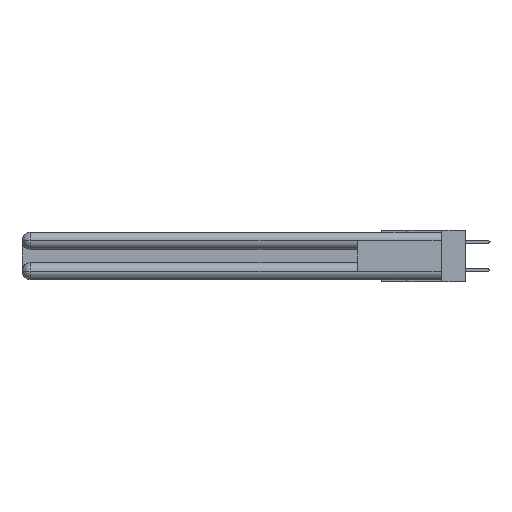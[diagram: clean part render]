
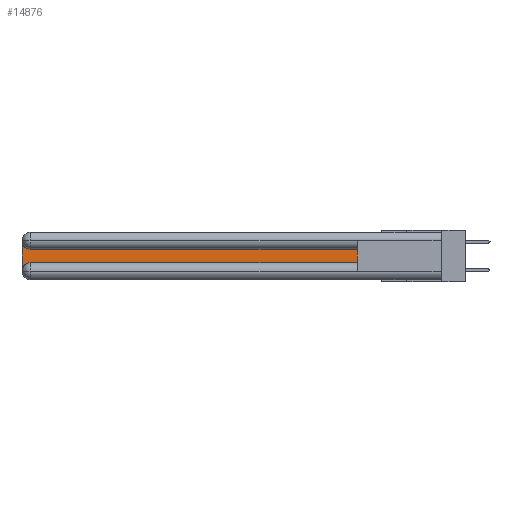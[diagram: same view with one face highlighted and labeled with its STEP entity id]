
A CAD part, left-side view. The second image highlights one B-rep face of the part: STEP entity #14876.
In plain terms, the highlighted planar face has unit normal (-1, 0, 0).
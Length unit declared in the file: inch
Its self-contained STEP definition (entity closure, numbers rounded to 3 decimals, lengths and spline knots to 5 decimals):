
#285 = ORIENTED_EDGE ( 'NONE', *, *, #8577, .T. ) ;
#614 = LINE ( 'NONE', #4832, #23441 ) ;
#1921 = CARTESIAN_POINT ( 'NONE',  ( 0.075, 0.6, -0.2175 ) ) ;
#2613 = VERTEX_POINT ( 'NONE', #20632 ) ;
#2625 = EDGE_CURVE ( 'NONE', #20399, #27930, #19876, .T. ) ;
#2728 = VECTOR ( 'NONE', #16100, 39.37008 ) ;
#3406 = LINE ( 'NONE', #16903, #12643 ) ;
#3561 = CARTESIAN_POINT ( 'NONE',  ( 0.075, 3., -0.2775 ) ) ;
#3810 = LINE ( 'NONE', #11492, #13066 ) ;
#4277 = DIRECTION ( 'NONE',  ( 0., 0., -1. ) ) ;
#4576 = CARTESIAN_POINT ( 'NONE',  ( 0.075, 2.94, -0.1225 ) ) ;
#4832 = CARTESIAN_POINT ( 'NONE',  ( 0.075, 3., -0.2175 ) ) ;
#4980 = DIRECTION ( 'NONE',  ( 0., 1., 0. ) ) ;
#5067 = DIRECTION ( 'NONE',  ( 0., 0., -1. ) ) ;
#5447 = LINE ( 'NONE', #9515, #2728 ) ;
#8577 = EDGE_CURVE ( 'NONE', #11617, #14855, #5447, .T. ) ;
#9515 = CARTESIAN_POINT ( 'NONE',  ( 0.075, 0.6, -0.2175 ) ) ;
#10604 = ORIENTED_EDGE ( 'NONE', *, *, #13892, .T. ) ;
#11492 = CARTESIAN_POINT ( 'NONE',  ( 0.075, 0.6, -0.1225 ) ) ;
#11617 = VERTEX_POINT ( 'NONE', #28042 ) ;
#12643 = VECTOR ( 'NONE', #14900, 39.37008 ) ;
#13066 = VECTOR ( 'NONE', #4980, 39.37008 ) ;
#13412 = ORIENTED_EDGE ( 'NONE', *, *, #23683, .T. ) ;
#13892 = EDGE_CURVE ( 'NONE', #14855, #2613, #3406, .T. ) ;
#14855 = VERTEX_POINT ( 'NONE', #1921 ) ;
#14876 = ADVANCED_FACE ( 'NONE', ( #20100 ), #21933, .F. ) ;
#14900 = DIRECTION ( 'NONE',  ( 0., 0., 1. ) ) ;
#15881 = DIRECTION ( 'NONE',  ( 1., 0., 0. ) ) ;
#15980 = CARTESIAN_POINT ( 'NONE',  ( 0.075, 2.94, -0.2775 ) ) ;
#16100 = DIRECTION ( 'NONE',  ( 0., -1., 0. ) ) ;
#16671 = ORIENTED_EDGE ( 'NONE', *, *, #2625, .T. ) ;
#16903 = CARTESIAN_POINT ( 'NONE',  ( 0.075, 0.6, -0.2175 ) ) ;
#17474 = CARTESIAN_POINT ( 'NONE',  ( 0.075, 3., -0.1225 ) ) ;
#17581 = EDGE_CURVE ( 'NONE', #21963, #11617, #25026, .T. ) ;
#17650 = EDGE_CURVE ( 'NONE', #2613, #20399, #3810, .T. ) ;
#18862 = ORIENTED_EDGE ( 'NONE', *, *, #17650, .T. ) ;
#19005 = AXIS2_PLACEMENT_3D ( 'NONE', #15980, #15881, #5067 ) ;
#19876 = CIRCLE ( 'NONE', #26427, 0.06 ) ;
#20100 = FACE_OUTER_BOUND ( 'NONE', #24350, .T. ) ;
#20399 = VERTEX_POINT ( 'NONE', #4576 ) ;
#20632 = CARTESIAN_POINT ( 'NONE',  ( 0.075, 0.6, -0.1225 ) ) ;
#21182 = CARTESIAN_POINT ( 'NONE',  ( 0.075, 2.94, -0.0625 ) ) ;
#21277 = DIRECTION ( 'NONE',  ( 1., 0., 0. ) ) ;
#21933 = PLANE ( 'NONE',  #25489 ) ;
#21963 = VERTEX_POINT ( 'NONE', #3561 ) ;
#23441 = VECTOR ( 'NONE', #24624, 39.37008 ) ;
#23683 = EDGE_CURVE ( 'NONE', #27930, #21963, #614, .T. ) ;
#23802 = ORIENTED_EDGE ( 'NONE', *, *, #17581, .T. ) ;
#24153 = DIRECTION ( 'NONE',  ( 1., 0., 0. ) ) ;
#24350 = EDGE_LOOP ( 'NONE', ( #18862, #16671, #13412, #23802, #285, #10604 ) ) ;
#24624 = DIRECTION ( 'NONE',  ( 0., 0., -1. ) ) ;
#25026 = CIRCLE ( 'NONE', #19005, 0.06 ) ;
#25489 = AXIS2_PLACEMENT_3D ( 'NONE', #17474, #24153, #4277 ) ;
#25722 = DIRECTION ( 'NONE',  ( 0., 0., -1. ) ) ;
#26427 = AXIS2_PLACEMENT_3D ( 'NONE', #21182, #21277, #25722 ) ;
#27930 = VERTEX_POINT ( 'NONE', #27972 ) ;
#27972 = CARTESIAN_POINT ( 'NONE',  ( 0.075, 3., -0.0625 ) ) ;
#28042 = CARTESIAN_POINT ( 'NONE',  ( 0.075, 2.94, -0.2175 ) ) ;
